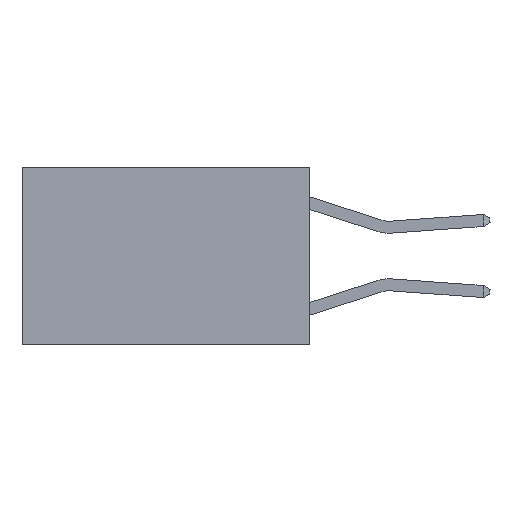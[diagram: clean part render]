
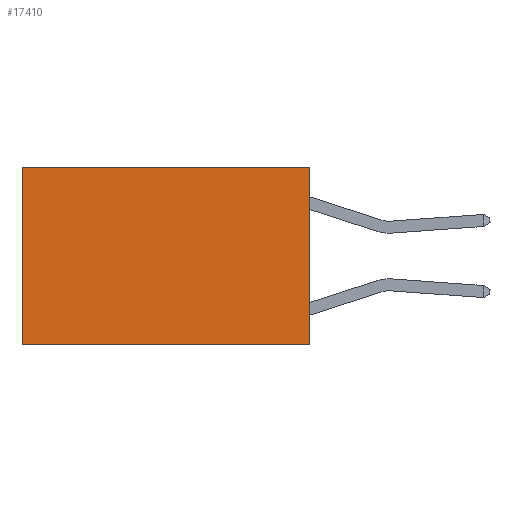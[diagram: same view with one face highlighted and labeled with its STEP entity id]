
A CAD part, left-side view. The second image highlights one B-rep face of the part: STEP entity #17410.
In plain terms, the highlighted planar face has unit normal (-1, 0, 0).
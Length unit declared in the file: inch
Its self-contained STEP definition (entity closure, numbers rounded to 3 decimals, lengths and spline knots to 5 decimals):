
#907 = VECTOR ( 'NONE', #19848, 39.37008 ) ;
#1290 = EDGE_CURVE ( 'NONE', #21704, #10785, #19137, .T. ) ;
#1343 = LINE ( 'NONE', #3605, #13773 ) ;
#2469 = ORIENTED_EDGE ( 'NONE', *, *, #20559, .T. ) ;
#3524 = CARTESIAN_POINT ( 'NONE',  ( 0.2625, 0.6, 0. ) ) ;
#3605 = CARTESIAN_POINT ( 'NONE',  ( 0.2625, 0.6, 0. ) ) ;
#4212 = ORIENTED_EDGE ( 'NONE', *, *, #17560, .T. ) ;
#4881 = DIRECTION ( 'NONE',  ( 0., 1., 0. ) ) ;
#6042 = VECTOR ( 'NONE', #13516, 39.37008 ) ;
#6450 = ORIENTED_EDGE ( 'NONE', *, *, #1290, .F. ) ;
#6935 = ORIENTED_EDGE ( 'NONE', *, *, #21140, .F. ) ;
#7769 = EDGE_LOOP ( 'NONE', ( #4212, #6935, #6450, #2469 ) ) ;
#8059 = CARTESIAN_POINT ( 'NONE',  ( 0.2625, 0., 0. ) ) ;
#8136 = CARTESIAN_POINT ( 'NONE',  ( 0.2625, 0., 0. ) ) ;
#8178 = DIRECTION ( 'NONE',  ( 0., 0., -1. ) ) ;
#8780 = AXIS2_PLACEMENT_3D ( 'NONE', #8059, #10296, #8178 ) ;
#9080 = LINE ( 'NONE', #23336, #907 ) ;
#9841 = PLANE ( 'NONE',  #8780 ) ;
#9953 = FACE_OUTER_BOUND ( 'NONE', #7769, .T. ) ;
#10296 = DIRECTION ( 'NONE',  ( 1., 0., 0. ) ) ;
#10610 = LINE ( 'NONE', #17667, #23059 ) ;
#10785 = VERTEX_POINT ( 'NONE', #14167 ) ;
#11339 = CARTESIAN_POINT ( 'NONE',  ( 0.2625, 0.6, -0.37 ) ) ;
#11454 = CARTESIAN_POINT ( 'NONE',  ( 0.2625, 0., 0. ) ) ;
#12687 = DIRECTION ( 'NONE',  ( 0., 0., -1. ) ) ;
#13153 = VERTEX_POINT ( 'NONE', #3524 ) ;
#13516 = DIRECTION ( 'NONE',  ( 0., 0., -1. ) ) ;
#13773 = VECTOR ( 'NONE', #12687, 39.37008 ) ;
#14167 = CARTESIAN_POINT ( 'NONE',  ( 0.2625, 0., -0.37 ) ) ;
#17410 = ADVANCED_FACE ( 'NONE', ( #9953 ), #9841, .F. ) ;
#17560 = EDGE_CURVE ( 'NONE', #13153, #21755, #1343, .T. ) ;
#17667 = CARTESIAN_POINT ( 'NONE',  ( 0.2625, 0., -0.37 ) ) ;
#19137 = LINE ( 'NONE', #8136, #6042 ) ;
#19848 = DIRECTION ( 'NONE',  ( 0., 1., 0. ) ) ;
#20559 = EDGE_CURVE ( 'NONE', #21704, #13153, #9080, .T. ) ;
#21140 = EDGE_CURVE ( 'NONE', #10785, #21755, #10610, .T. ) ;
#21704 = VERTEX_POINT ( 'NONE', #11454 ) ;
#21755 = VERTEX_POINT ( 'NONE', #11339 ) ;
#23059 = VECTOR ( 'NONE', #4881, 39.37008 ) ;
#23336 = CARTESIAN_POINT ( 'NONE',  ( 0.2625, 0., 0. ) ) ;
